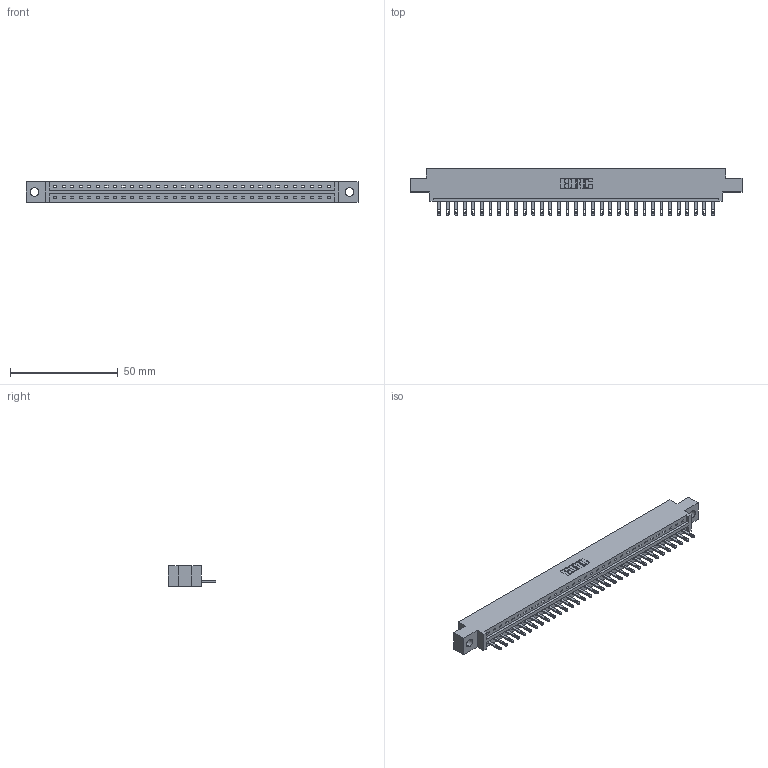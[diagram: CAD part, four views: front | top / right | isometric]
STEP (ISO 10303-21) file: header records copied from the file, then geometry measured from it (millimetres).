
FILE_DESCRIPTION (( 'STEP AP203' ), '1' );
FILE_NAME ('337-033-500-604.STEP', '2018-08-07T07:58:47', ( '' ), ( '' ), 'SwSTEP 2.0', 'SolidWorks 2016', '' );
FILE_SCHEMA (( 'CONFIG_CONTROL_DESIGN' ));
Length unit declared in the file: inch
Products named in the file (3): 337 Part_0.170 Offset - 0.156 Dia-TH; 345-292-001_345-293-100; 337-033-500-604
Assembly tree (34 placements, depth 2):
  337-033-500-604
    337 Part_0.170 Offset - 0.156 Dia-TH
    345-292-001_345-293-100  x33
Bounding box: 153.77 x 21.85 x 9.4 mm (x, y, z)
Volume: 15684.4 mm3; surface area: 16126.3 mm2
Topology: 34 solids, 34 shells, 2032 faces, 6263 edges, 4174 vertices
Faces by surface type: plane 1394, cylinder 638
Entity records: 25759 total; most frequent: CARTESIAN_POINT 4493, ORIENTED_EDGE 4462, DIRECTION 3801, EDGE_CURVE 2231, LINE 2099, VECTOR 2099, VERTEX_POINT 1486, AXIS2_PLACEMENT_3D 851
